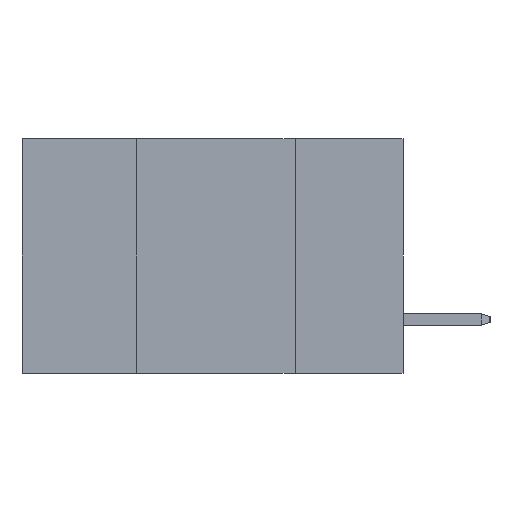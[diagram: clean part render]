
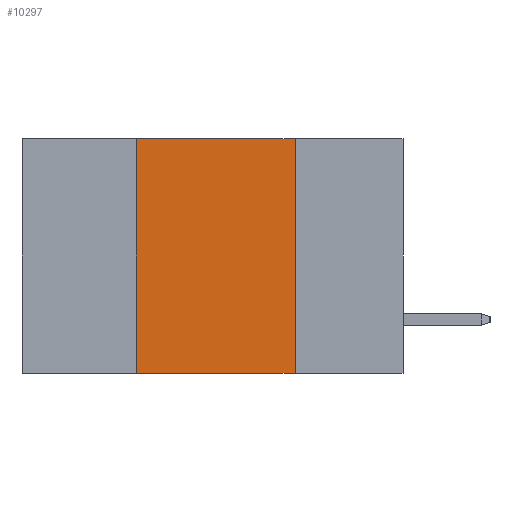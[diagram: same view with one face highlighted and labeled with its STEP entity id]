
A CAD part, left-side view. The second image highlights one B-rep face of the part: STEP entity #10297.
In plain terms, the highlighted planar face has unit normal (-1, 0, 0).
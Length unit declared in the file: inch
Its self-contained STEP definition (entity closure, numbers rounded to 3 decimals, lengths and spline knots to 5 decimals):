
#503 = ORIENTED_EDGE ( 'NONE', *, *, #7107, .F. ) ;
#1099 = VERTEX_POINT ( 'NONE', #9246 ) ;
#1454 = CARTESIAN_POINT ( 'NONE',  ( 0., 0.42, 0. ) ) ;
#1700 = CARTESIAN_POINT ( 'NONE',  ( 0., 0.42, -0.37 ) ) ;
#1831 = CARTESIAN_POINT ( 'NONE',  ( 0., 0.6, -0.37 ) ) ;
#2148 = CARTESIAN_POINT ( 'NONE',  ( 0., 0.6, 0. ) ) ;
#2223 = DIRECTION ( 'NONE',  ( 0., 0., 1. ) ) ;
#2496 = DIRECTION ( 'NONE',  ( 0., -1., 0. ) ) ;
#2659 = CARTESIAN_POINT ( 'NONE',  ( 0., 0.6, 0. ) ) ;
#2701 = EDGE_CURVE ( 'NONE', #1099, #3791, #14486, .T. ) ;
#3023 = LINE ( 'NONE', #1831, #9188 ) ;
#3106 = LINE ( 'NONE', #9473, #3761 ) ;
#3761 = VECTOR ( 'NONE', #2223, 39.37008 ) ;
#3791 = VERTEX_POINT ( 'NONE', #12223 ) ;
#4252 = EDGE_LOOP ( 'NONE', ( #7643, #7460, #503, #10709 ) ) ;
#4899 = LINE ( 'NONE', #2659, #7164 ) ;
#6352 = AXIS2_PLACEMENT_3D ( 'NONE', #2148, #7076, #11940 ) ;
#6889 = EDGE_CURVE ( 'NONE', #14982, #1099, #4899, .T. ) ;
#6928 = EDGE_CURVE ( 'NONE', #8343, #3791, #3023, .T. ) ;
#7076 = DIRECTION ( 'NONE',  ( 1., 0., 0. ) ) ;
#7107 = EDGE_CURVE ( 'NONE', #8343, #14982, #3106, .T. ) ;
#7164 = VECTOR ( 'NONE', #12363, 39.37008 ) ;
#7460 = ORIENTED_EDGE ( 'NONE', *, *, #6889, .F. ) ;
#7601 = VECTOR ( 'NONE', #13131, 39.37008 ) ;
#7643 = ORIENTED_EDGE ( 'NONE', *, *, #2701, .F. ) ;
#8343 = VERTEX_POINT ( 'NONE', #1700 ) ;
#9188 = VECTOR ( 'NONE', #2496, 39.37008 ) ;
#9246 = CARTESIAN_POINT ( 'NONE',  ( 0., 0.17, 0. ) ) ;
#9473 = CARTESIAN_POINT ( 'NONE',  ( 0., 0.42, 0. ) ) ;
#10297 = ADVANCED_FACE ( 'NONE', ( #15587 ), #13368, .F. ) ;
#10709 = ORIENTED_EDGE ( 'NONE', *, *, #6928, .T. ) ;
#11940 = DIRECTION ( 'NONE',  ( 0., 0., -1. ) ) ;
#12223 = CARTESIAN_POINT ( 'NONE',  ( 0., 0.17, -0.37 ) ) ;
#12363 = DIRECTION ( 'NONE',  ( 0., -1., 0. ) ) ;
#13131 = DIRECTION ( 'NONE',  ( 0., 0., -1. ) ) ;
#13296 = CARTESIAN_POINT ( 'NONE',  ( 0., 0.17, 0. ) ) ;
#13368 = PLANE ( 'NONE',  #6352 ) ;
#14486 = LINE ( 'NONE', #13296, #7601 ) ;
#14982 = VERTEX_POINT ( 'NONE', #1454 ) ;
#15587 = FACE_OUTER_BOUND ( 'NONE', #4252, .T. ) ;
